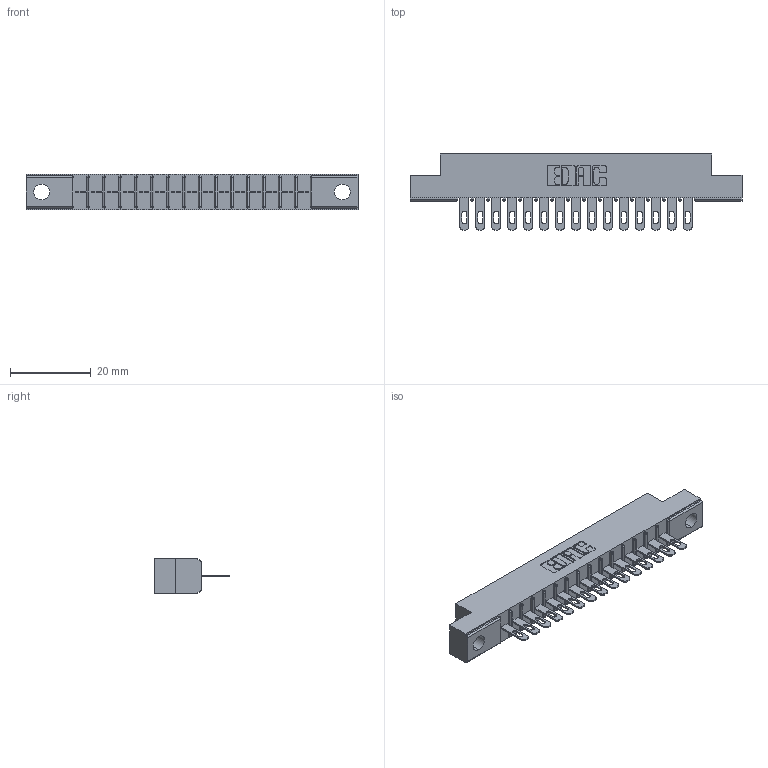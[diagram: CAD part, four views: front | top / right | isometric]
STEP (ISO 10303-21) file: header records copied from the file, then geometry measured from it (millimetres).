
FILE_DESCRIPTION (( 'STEP AP203' ), '1' );
FILE_NAME ('316-015-400-104.STEP', '2020-09-22T17:12:08', ( '' ), ( '' ), 'SwSTEP 2.0', 'SolidWorks 2020', '' );
FILE_SCHEMA (( 'CONFIG_CONTROL_DESIGN' ));
Length unit declared in the file: inch
Products named in the file (3): 316-015-400-104; 306 Part_.156 Dia; 306-290-001_100
Assembly tree (16 placements, depth 2):
  316-015-400-104
    306 Part_.156 Dia
    306-290-001_100  x15
Bounding box: 82.45 x 18.87 x 8.71 mm (x, y, z)
Volume: 5554.2 mm3; surface area: 8083.7 mm2
Topology: 16 solids, 16 shells, 1270 faces, 3577 edges, 2302 vertices
Faces by surface type: plane 832, cylinder 378, sphere 60
Entity records: 18068 total; most frequent: CARTESIAN_POINT 3034, ORIENTED_EDGE 3002, DIRECTION 2987, EDGE_CURVE 1501, VECTOR 1165, LINE 1165, VERTEX_POINT 958, AXIS2_PLACEMENT_3D 911
